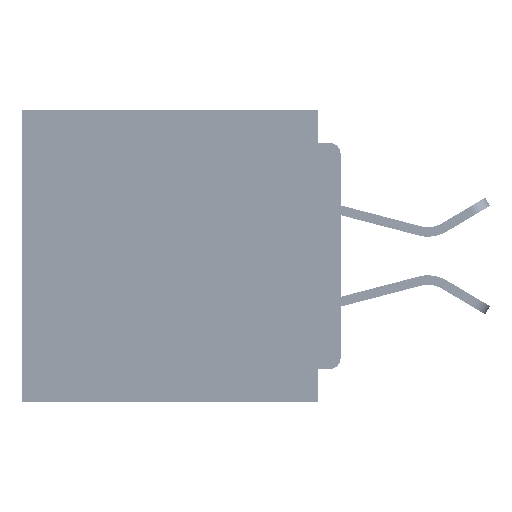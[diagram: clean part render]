
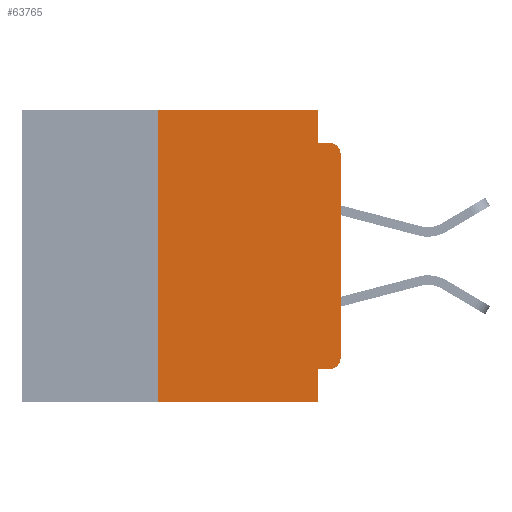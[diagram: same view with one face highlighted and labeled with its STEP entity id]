
A CAD part, left-side view. The second image highlights one B-rep face of the part: STEP entity #63765.
In plain terms, the highlighted planar face has unit normal (-1, 0, 0).
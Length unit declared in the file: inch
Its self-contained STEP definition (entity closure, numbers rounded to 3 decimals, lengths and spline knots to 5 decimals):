
#503 = LINE ( 'NONE', #41734, #52002 ) ;
#820 = DIRECTION ( 'NONE',  ( -1., 0., 0. ) ) ;
#1189 = VERTEX_POINT ( 'NONE', #59116 ) ;
#1265 = PLANE ( 'NONE',  #59404 ) ;
#1629 = DIRECTION ( 'NONE',  ( 0., -1., 0. ) ) ;
#3395 = CARTESIAN_POINT ( 'NONE',  ( 0., 0.25, 0. ) ) ;
#4151 = ORIENTED_EDGE ( 'NONE', *, *, #14598, .T. ) ;
#5766 = LINE ( 'NONE', #35298, #30777 ) ;
#7053 = EDGE_LOOP ( 'NONE', ( #16644, #30428, #8119, #49039, #21339, #9587, #4151, #14851, #26766, #24276 ) ) ;
#8119 = ORIENTED_EDGE ( 'NONE', *, *, #50718, .F. ) ;
#8470 = CARTESIAN_POINT ( 'NONE',  ( 0., 0.015, -0.045 ) ) ;
#9273 = VERTEX_POINT ( 'NONE', #15534 ) ;
#9353 = DIRECTION ( 'NONE',  ( 0., 0., -1. ) ) ;
#9587 = ORIENTED_EDGE ( 'NONE', *, *, #18619, .F. ) ;
#10224 = CARTESIAN_POINT ( 'NONE',  ( 0., 0., -0.06 ) ) ;
#10323 = VECTOR ( 'NONE', #23420, 39.37008 ) ;
#11357 = DIRECTION ( 'NONE',  ( 0., 0., -1. ) ) ;
#12030 = LINE ( 'NONE', #44256, #51756 ) ;
#12134 = VERTEX_POINT ( 'NONE', #3395 ) ;
#13348 = CARTESIAN_POINT ( 'NONE',  ( 0., 0.015, -0.06 ) ) ;
#14598 = EDGE_CURVE ( 'NONE', #58469, #31175, #5766, .T. ) ;
#14786 = EDGE_CURVE ( 'NONE', #12134, #46458, #47875, .T. ) ;
#14851 = ORIENTED_EDGE ( 'NONE', *, *, #38532, .F. ) ;
#15534 = CARTESIAN_POINT ( 'NONE',  ( 0., 0.031, -0.045 ) ) ;
#16534 = VECTOR ( 'NONE', #17012, 39.37008 ) ;
#16644 = ORIENTED_EDGE ( 'NONE', *, *, #21171, .T. ) ;
#16682 = CARTESIAN_POINT ( 'NONE',  ( 0., 0.031, -0.4 ) ) ;
#17012 = DIRECTION ( 'NONE',  ( 0., 1., 0. ) ) ;
#17507 = VECTOR ( 'NONE', #25763, 39.37008 ) ;
#18384 = DIRECTION ( 'NONE',  ( 0., 0., -1. ) ) ;
#18619 = EDGE_CURVE ( 'NONE', #58469, #12134, #503, .T. ) ;
#19736 = CIRCLE ( 'NONE', #32168, 0.015 ) ;
#21171 = EDGE_CURVE ( 'NONE', #52286, #53785, #36862, .T. ) ;
#21339 = ORIENTED_EDGE ( 'NONE', *, *, #14786, .F. ) ;
#21920 = DIRECTION ( 'NONE',  ( 0., 0., 1. ) ) ;
#23420 = DIRECTION ( 'NONE',  ( 0., 0., 1. ) ) ;
#24276 = ORIENTED_EDGE ( 'NONE', *, *, #46932, .T. ) ;
#25763 = DIRECTION ( 'NONE',  ( 0., -1., 0. ) ) ;
#26766 = ORIENTED_EDGE ( 'NONE', *, *, #45696, .F. ) ;
#29788 = LINE ( 'NONE', #51843, #16534 ) ;
#30428 = ORIENTED_EDGE ( 'NONE', *, *, #45230, .T. ) ;
#30764 = CARTESIAN_POINT ( 'NONE',  ( 0., 0.015, -0.34 ) ) ;
#30777 = VECTOR ( 'NONE', #40308, 39.37008 ) ;
#31175 = VERTEX_POINT ( 'NONE', #16682 ) ;
#32168 = AXIS2_PLACEMENT_3D ( 'NONE', #13348, #48188, #18384 ) ;
#32327 = LINE ( 'NONE', #60609, #17507 ) ;
#33835 = VERTEX_POINT ( 'NONE', #53492 ) ;
#35298 = CARTESIAN_POINT ( 'NONE',  ( 0., 0.437, -0.4 ) ) ;
#35772 = DIRECTION ( 'NONE',  ( 0., 0., -1. ) ) ;
#36862 = LINE ( 'NONE', #58239, #10323 ) ;
#37427 = CIRCLE ( 'NONE', #59330, 0.015 ) ;
#38532 = EDGE_CURVE ( 'NONE', #33835, #31175, #39000, .T. ) ;
#39000 = LINE ( 'NONE', #44790, #49111 ) ;
#40308 = DIRECTION ( 'NONE',  ( 0., -1., 0. ) ) ;
#41213 = DIRECTION ( 'NONE',  ( 1., 0., 0. ) ) ;
#41572 = CARTESIAN_POINT ( 'NONE',  ( 0., 0.437, 0. ) ) ;
#41734 = CARTESIAN_POINT ( 'NONE',  ( 0., 0.25, -0.4 ) ) ;
#42001 = CARTESIAN_POINT ( 'NONE',  ( 0., 0., -0.34 ) ) ;
#44256 = CARTESIAN_POINT ( 'NONE',  ( 0., 0.031, 0. ) ) ;
#44790 = CARTESIAN_POINT ( 'NONE',  ( 0., 0.031, -0.4 ) ) ;
#45230 = EDGE_CURVE ( 'NONE', #53785, #64045, #19736, .T. ) ;
#45296 = FACE_OUTER_BOUND ( 'NONE', #7053, .T. ) ;
#45696 = EDGE_CURVE ( 'NONE', #1189, #33835, #29788, .T. ) ;
#46339 = VECTOR ( 'NONE', #1629, 39.37008 ) ;
#46458 = VERTEX_POINT ( 'NONE', #51698 ) ;
#46932 = EDGE_CURVE ( 'NONE', #1189, #52286, #37427, .T. ) ;
#47875 = LINE ( 'NONE', #41572, #46339 ) ;
#48188 = DIRECTION ( 'NONE',  ( -1., 0., 0. ) ) ;
#49039 = ORIENTED_EDGE ( 'NONE', *, *, #55101, .F. ) ;
#49111 = VECTOR ( 'NONE', #49762, 39.37008 ) ;
#49762 = DIRECTION ( 'NONE',  ( 0., 0., -1. ) ) ;
#50718 = EDGE_CURVE ( 'NONE', #9273, #64045, #32327, .T. ) ;
#51407 = CARTESIAN_POINT ( 'NONE',  ( 0., 0.25, -0.4 ) ) ;
#51698 = CARTESIAN_POINT ( 'NONE',  ( 0., 0.031, 0. ) ) ;
#51756 = VECTOR ( 'NONE', #9353, 39.37008 ) ;
#51843 = CARTESIAN_POINT ( 'NONE',  ( 0., 0., -0.355 ) ) ;
#52002 = VECTOR ( 'NONE', #21920, 39.37008 ) ;
#52286 = VERTEX_POINT ( 'NONE', #42001 ) ;
#53492 = CARTESIAN_POINT ( 'NONE',  ( 0., 0.031, -0.355 ) ) ;
#53785 = VERTEX_POINT ( 'NONE', #10224 ) ;
#55101 = EDGE_CURVE ( 'NONE', #46458, #9273, #12030, .T. ) ;
#56003 = CARTESIAN_POINT ( 'NONE',  ( 0., 0.437, 0. ) ) ;
#58239 = CARTESIAN_POINT ( 'NONE',  ( 0., 0., 0. ) ) ;
#58469 = VERTEX_POINT ( 'NONE', #51407 ) ;
#59116 = CARTESIAN_POINT ( 'NONE',  ( 0., 0.015, -0.355 ) ) ;
#59330 = AXIS2_PLACEMENT_3D ( 'NONE', #30764, #820, #35772 ) ;
#59404 = AXIS2_PLACEMENT_3D ( 'NONE', #56003, #41213, #11357 ) ;
#60609 = CARTESIAN_POINT ( 'NONE',  ( 0., 0., -0.045 ) ) ;
#63765 = ADVANCED_FACE ( 'NONE', ( #45296 ), #1265, .F. ) ;
#64045 = VERTEX_POINT ( 'NONE', #8470 ) ;
